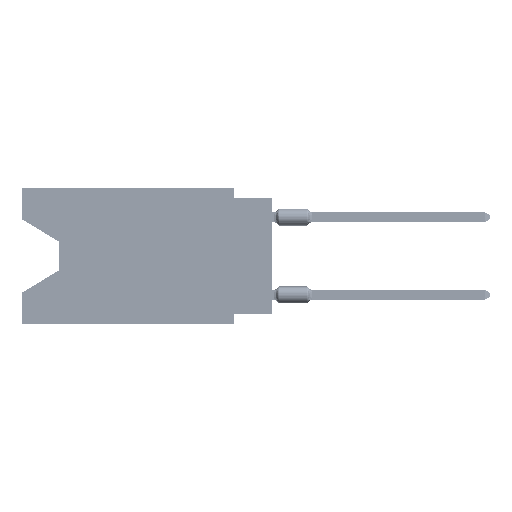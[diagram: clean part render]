
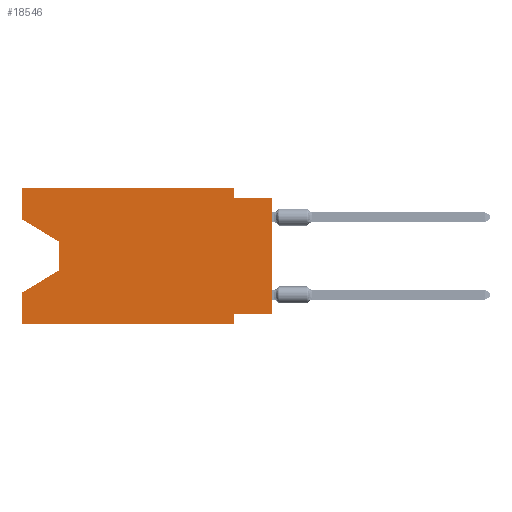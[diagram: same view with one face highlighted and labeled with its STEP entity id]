
A CAD part, left-side view. The second image highlights one B-rep face of the part: STEP entity #18546.
In plain terms, the highlighted planar face has unit normal (-1, 0, 0).
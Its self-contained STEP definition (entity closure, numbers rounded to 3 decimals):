
#475 = DIRECTION ( 'NONE',  ( 1., 0., 0. ) ) ;
#1135 = VERTEX_POINT ( 'NONE', #37705 ) ;
#1172 = LINE ( 'NONE', #26522, #17746 ) ;
#1307 = VECTOR ( 'NONE', #61352, 1000. ) ;
#2088 = VERTEX_POINT ( 'NONE', #6935 ) ;
#2889 = EDGE_CURVE ( 'NONE', #2088, #28315, #41043, .T. ) ;
#3946 = VECTOR ( 'NONE', #63856, 1000. ) ;
#4107 = LINE ( 'NONE', #82176, #31399 ) ;
#4311 = CARTESIAN_POINT ( 'NONE',  ( 0., 0., 0. ) ) ;
#4442 = CARTESIAN_POINT ( 'NONE',  ( 0., 13.97, -5.385 ) ) ;
#4480 = CARTESIAN_POINT ( 'NONE',  ( 0., 2.54, -8.89 ) ) ;
#4676 = ORIENTED_EDGE ( 'NONE', *, *, #77680, .F. ) ;
#5622 = CARTESIAN_POINT ( 'NONE',  ( 0., 16.383, 0. ) ) ;
#6056 = EDGE_CURVE ( 'NONE', #78945, #1135, #70204, .T. ) ;
#6150 = VECTOR ( 'NONE', #24851, 1000. ) ;
#6736 = DIRECTION ( 'NONE',  ( 0., 0., 1. ) ) ;
#6935 = CARTESIAN_POINT ( 'NONE',  ( 0., 2.54, -0.635 ) ) ;
#7859 = LINE ( 'NONE', #12694, #27341 ) ;
#7904 = CARTESIAN_POINT ( 'NONE',  ( 0., 0., -0.635 ) ) ;
#8151 = CARTESIAN_POINT ( 'NONE',  ( 0., 0., -8.255 ) ) ;
#8916 = VERTEX_POINT ( 'NONE', #28054 ) ;
#11737 = LINE ( 'NONE', #5622, #6150 ) ;
#12088 = EDGE_CURVE ( 'NONE', #32814, #78945, #7859, .T. ) ;
#12694 = CARTESIAN_POINT ( 'NONE',  ( 0., 16.383, -2.038 ) ) ;
#13588 = VECTOR ( 'NONE', #6736, 1000. ) ;
#13875 = EDGE_CURVE ( 'NONE', #32814, #59295, #63107, .T. ) ;
#14353 = VERTEX_POINT ( 'NONE', #51220 ) ;
#15736 = ORIENTED_EDGE ( 'NONE', *, *, #16601, .F. ) ;
#16391 = EDGE_CURVE ( 'NONE', #18455, #28315, #64065, .T. ) ;
#16601 = EDGE_CURVE ( 'NONE', #14353, #2088, #82603, .T. ) ;
#17468 = ORIENTED_EDGE ( 'NONE', *, *, #6056, .T. ) ;
#17746 = VECTOR ( 'NONE', #27802, 1000. ) ;
#18455 = VERTEX_POINT ( 'NONE', #54526 ) ;
#18546 = ADVANCED_FACE ( 'NONE', ( #34071 ), #26689, .F. ) ;
#21249 = LINE ( 'NONE', #8151, #1307 ) ;
#22888 = DIRECTION ( 'NONE',  ( 0., -1., 0. ) ) ;
#23057 = EDGE_CURVE ( 'NONE', #59295, #14353, #11737, .T. ) ;
#23770 = CARTESIAN_POINT ( 'NONE',  ( 0., 2.54, 0. ) ) ;
#24851 = DIRECTION ( 'NONE',  ( 0., -1., 0. ) ) ;
#26387 = CARTESIAN_POINT ( 'NONE',  ( 0., 16.383, 0. ) ) ;
#26522 = CARTESIAN_POINT ( 'NONE',  ( 0., 2.54, -8.89 ) ) ;
#26689 = PLANE ( 'NONE',  #66711 ) ;
#27341 = VECTOR ( 'NONE', #79817, 1000. ) ;
#27802 = DIRECTION ( 'NONE',  ( 0., 0., -1. ) ) ;
#28054 = CARTESIAN_POINT ( 'NONE',  ( 0., 16.383, -8.89 ) ) ;
#28315 = VERTEX_POINT ( 'NONE', #42362 ) ;
#30938 = DIRECTION ( 'NONE',  ( 0., 0., 1. ) ) ;
#31399 = VECTOR ( 'NONE', #22888, 1000. ) ;
#31678 = ORIENTED_EDGE ( 'NONE', *, *, #62301, .T. ) ;
#32814 = VERTEX_POINT ( 'NONE', #44522 ) ;
#33702 = CARTESIAN_POINT ( 'NONE',  ( 0., 13.97, -3.505 ) ) ;
#33730 = ORIENTED_EDGE ( 'NONE', *, *, #43896, .F. ) ;
#34026 = ORIENTED_EDGE ( 'NONE', *, *, #2889, .F. ) ;
#34071 = FACE_OUTER_BOUND ( 'NONE', #81323, .T. ) ;
#34816 = DIRECTION ( 'NONE',  ( 0., 0., 1. ) ) ;
#35958 = CARTESIAN_POINT ( 'NONE',  ( 0., 16.383, -6.852 ) ) ;
#37606 = LINE ( 'NONE', #4442, #83090 ) ;
#37705 = CARTESIAN_POINT ( 'NONE',  ( 0., 13.97, -5.385 ) ) ;
#39893 = VECTOR ( 'NONE', #34816, 1000. ) ;
#40732 = ORIENTED_EDGE ( 'NONE', *, *, #60626, .T. ) ;
#41043 = LINE ( 'NONE', #7904, #47337 ) ;
#42362 = CARTESIAN_POINT ( 'NONE',  ( 0., 0., -0.635 ) ) ;
#42421 = ORIENTED_EDGE ( 'NONE', *, *, #12088, .T. ) ;
#43896 = EDGE_CURVE ( 'NONE', #85138, #57058, #1172, .T. ) ;
#44522 = CARTESIAN_POINT ( 'NONE',  ( 0., 16.383, -2.038 ) ) ;
#45113 = LINE ( 'NONE', #26387, #13588 ) ;
#46712 = DIRECTION ( 'NONE',  ( 0., 0., -1. ) ) ;
#47337 = VECTOR ( 'NONE', #54119, 1000. ) ;
#51220 = CARTESIAN_POINT ( 'NONE',  ( 0., 2.54, 0. ) ) ;
#53240 = CARTESIAN_POINT ( 'NONE',  ( 0., 16.383, 0. ) ) ;
#54119 = DIRECTION ( 'NONE',  ( 0., -1., 0. ) ) ;
#54526 = CARTESIAN_POINT ( 'NONE',  ( 0., 0., -8.255 ) ) ;
#55136 = CARTESIAN_POINT ( 'NONE',  ( 0., 16.383, 0. ) ) ;
#56922 = ORIENTED_EDGE ( 'NONE', *, *, #13875, .F. ) ;
#57058 = VERTEX_POINT ( 'NONE', #4480 ) ;
#59295 = VERTEX_POINT ( 'NONE', #55136 ) ;
#60179 = VECTOR ( 'NONE', #62797, 1000. ) ;
#60626 = EDGE_CURVE ( 'NONE', #8916, #57058, #4107, .T. ) ;
#61352 = DIRECTION ( 'NONE',  ( 0., 1., 0. ) ) ;
#62301 = EDGE_CURVE ( 'NONE', #1135, #81692, #37606, .T. ) ;
#62458 = VECTOR ( 'NONE', #30938, 1000. ) ;
#62797 = DIRECTION ( 'NONE',  ( 0., 0., -1. ) ) ;
#63107 = LINE ( 'NONE', #74893, #39893 ) ;
#63856 = DIRECTION ( 'NONE',  ( 0., 0., -1. ) ) ;
#64065 = LINE ( 'NONE', #4311, #62458 ) ;
#66257 = ORIENTED_EDGE ( 'NONE', *, *, #16391, .T. ) ;
#66711 = AXIS2_PLACEMENT_3D ( 'NONE', #53240, #475, #46712 ) ;
#70204 = LINE ( 'NONE', #83721, #60179 ) ;
#74893 = CARTESIAN_POINT ( 'NONE',  ( 0., 16.383, 0. ) ) ;
#75015 = EDGE_CURVE ( 'NONE', #8916, #81692, #45113, .T. ) ;
#75575 = CARTESIAN_POINT ( 'NONE',  ( 0., 2.54, -8.255 ) ) ;
#77680 = EDGE_CURVE ( 'NONE', #18455, #85138, #21249, .T. ) ;
#77824 = ORIENTED_EDGE ( 'NONE', *, *, #75015, .F. ) ;
#78945 = VERTEX_POINT ( 'NONE', #33702 ) ;
#79817 = DIRECTION ( 'NONE',  ( 0., -0.855, -0.519 ) ) ;
#81323 = EDGE_LOOP ( 'NONE', ( #42421, #17468, #31678, #77824, #40732, #33730, #4676, #66257, #34026, #15736, #82298, #56922 ) ) ;
#81692 = VERTEX_POINT ( 'NONE', #35958 ) ;
#82083 = DIRECTION ( 'NONE',  ( 0., 0.855, -0.519 ) ) ;
#82176 = CARTESIAN_POINT ( 'NONE',  ( 0., 16.383, -8.89 ) ) ;
#82298 = ORIENTED_EDGE ( 'NONE', *, *, #23057, .F. ) ;
#82603 = LINE ( 'NONE', #23770, #3946 ) ;
#83090 = VECTOR ( 'NONE', #82083, 1000. ) ;
#83721 = CARTESIAN_POINT ( 'NONE',  ( 0., 13.97, -3.505 ) ) ;
#85138 = VERTEX_POINT ( 'NONE', #75575 ) ;
